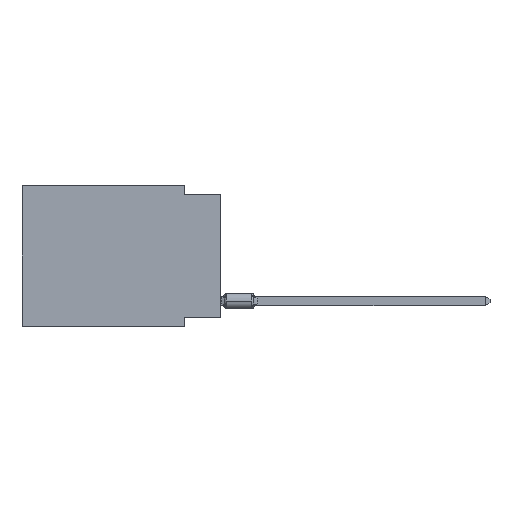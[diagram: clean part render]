
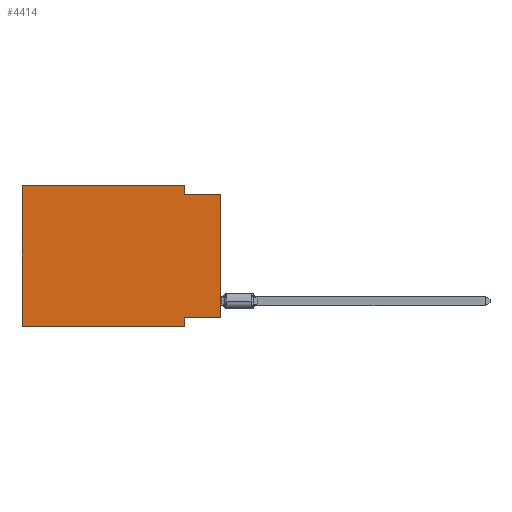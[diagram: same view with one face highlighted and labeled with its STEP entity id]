
A CAD part, left-side view. The second image highlights one B-rep face of the part: STEP entity #4414.
In plain terms, the highlighted planar face has unit normal (-1, 0, 0).
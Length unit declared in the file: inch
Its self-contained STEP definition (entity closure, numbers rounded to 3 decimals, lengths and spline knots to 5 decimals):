
#232 = DIRECTION ( 'NONE',  ( 0., -1., 0. ) ) ;
#452 = ORIENTED_EDGE ( 'NONE', *, *, #15030, .F. ) ;
#1070 = CARTESIAN_POINT ( 'NONE',  ( 0., 0.1, -0.39 ) ) ;
#1318 = LINE ( 'NONE', #1070, #5441 ) ;
#1820 = ORIENTED_EDGE ( 'NONE', *, *, #14614, .F. ) ;
#2452 = CARTESIAN_POINT ( 'NONE',  ( 0., 0., -0.025 ) ) ;
#2698 = LINE ( 'NONE', #4498, #14170 ) ;
#2872 = EDGE_CURVE ( 'NONE', #19427, #13744, #1318, .T. ) ;
#3164 = VECTOR ( 'NONE', #232, 39.37008 ) ;
#3829 = LINE ( 'NONE', #13427, #3164 ) ;
#4414 = ADVANCED_FACE ( 'NONE', ( #11755 ), #19069, .F. ) ;
#4498 = CARTESIAN_POINT ( 'NONE',  ( 0., 0.1, 0. ) ) ;
#4780 = CARTESIAN_POINT ( 'NONE',  ( 0., 0.55, 0. ) ) ;
#4867 = CARTESIAN_POINT ( 'NONE',  ( 0., 0.1, -0.39 ) ) ;
#5154 = EDGE_CURVE ( 'NONE', #9182, #17868, #16870, .T. ) ;
#5441 = VECTOR ( 'NONE', #8392, 39.37008 ) ;
#7120 = ORIENTED_EDGE ( 'NONE', *, *, #2872, .F. ) ;
#8354 = VECTOR ( 'NONE', #10966, 39.37008 ) ;
#8392 = DIRECTION ( 'NONE',  ( 0., 0., -1. ) ) ;
#9182 = VERTEX_POINT ( 'NONE', #14489 ) ;
#9201 = VECTOR ( 'NONE', #18908, 39.37008 ) ;
#9592 = VERTEX_POINT ( 'NONE', #16276 ) ;
#9670 = CARTESIAN_POINT ( 'NONE',  ( 0., 0., 0. ) ) ;
#10638 = EDGE_LOOP ( 'NONE', ( #14295, #13330, #23517, #16822, #1820, #18692, #7120, #452 ) ) ;
#10966 = DIRECTION ( 'NONE',  ( 0., 0., 1. ) ) ;
#11065 = VECTOR ( 'NONE', #11390, 39.37008 ) ;
#11390 = DIRECTION ( 'NONE',  ( 0., 1., 0. ) ) ;
#11427 = EDGE_CURVE ( 'NONE', #9592, #13744, #3829, .T. ) ;
#11755 = FACE_OUTER_BOUND ( 'NONE', #10638, .T. ) ;
#11759 = EDGE_CURVE ( 'NONE', #23703, #17868, #22747, .T. ) ;
#11925 = CARTESIAN_POINT ( 'NONE',  ( 0., 0., -0.025 ) ) ;
#12008 = VERTEX_POINT ( 'NONE', #16710 ) ;
#12633 = LINE ( 'NONE', #16476, #8354 ) ;
#12945 = CARTESIAN_POINT ( 'NONE',  ( 0., 0.55, 0. ) ) ;
#13330 = ORIENTED_EDGE ( 'NONE', *, *, #11759, .F. ) ;
#13383 = DIRECTION ( 'NONE',  ( 0., 0., -1. ) ) ;
#13427 = CARTESIAN_POINT ( 'NONE',  ( 0., 0.55, -0.39 ) ) ;
#13744 = VERTEX_POINT ( 'NONE', #4867 ) ;
#14131 = DIRECTION ( 'NONE',  ( 1., 0., 0. ) ) ;
#14170 = VECTOR ( 'NONE', #13383, 39.37008 ) ;
#14295 = ORIENTED_EDGE ( 'NONE', *, *, #5154, .T. ) ;
#14489 = CARTESIAN_POINT ( 'NONE',  ( 0., 0., -0.365 ) ) ;
#14614 = EDGE_CURVE ( 'NONE', #9592, #16806, #12633, .T. ) ;
#15030 = EDGE_CURVE ( 'NONE', #9182, #19427, #20242, .T. ) ;
#15275 = DIRECTION ( 'NONE',  ( 0., -1., 0. ) ) ;
#15423 = LINE ( 'NONE', #19474, #20814 ) ;
#16276 = CARTESIAN_POINT ( 'NONE',  ( 0., 0.55, -0.39 ) ) ;
#16476 = CARTESIAN_POINT ( 'NONE',  ( 0., 0.55, 0. ) ) ;
#16710 = CARTESIAN_POINT ( 'NONE',  ( 0., 0.1, 0. ) ) ;
#16788 = EDGE_CURVE ( 'NONE', #12008, #23703, #2698, .T. ) ;
#16806 = VERTEX_POINT ( 'NONE', #12945 ) ;
#16822 = ORIENTED_EDGE ( 'NONE', *, *, #22508, .F. ) ;
#16870 = LINE ( 'NONE', #9670, #9201 ) ;
#17354 = DIRECTION ( 'NONE',  ( 0., -1., 0. ) ) ;
#17868 = VERTEX_POINT ( 'NONE', #11925 ) ;
#18692 = ORIENTED_EDGE ( 'NONE', *, *, #11427, .T. ) ;
#18908 = DIRECTION ( 'NONE',  ( 0., 0., 1. ) ) ;
#19069 = PLANE ( 'NONE',  #21841 ) ;
#19427 = VERTEX_POINT ( 'NONE', #21134 ) ;
#19474 = CARTESIAN_POINT ( 'NONE',  ( 0., 0.55, 0. ) ) ;
#20242 = LINE ( 'NONE', #20377, #11065 ) ;
#20377 = CARTESIAN_POINT ( 'NONE',  ( 0., 0., -0.365 ) ) ;
#20814 = VECTOR ( 'NONE', #17354, 39.37008 ) ;
#21134 = CARTESIAN_POINT ( 'NONE',  ( 0., 0.1, -0.365 ) ) ;
#21456 = DIRECTION ( 'NONE',  ( 0., 0., -1. ) ) ;
#21841 = AXIS2_PLACEMENT_3D ( 'NONE', #4780, #14131, #21456 ) ;
#22508 = EDGE_CURVE ( 'NONE', #16806, #12008, #15423, .T. ) ;
#22747 = LINE ( 'NONE', #2452, #23111 ) ;
#23019 = CARTESIAN_POINT ( 'NONE',  ( 0., 0.1, -0.025 ) ) ;
#23111 = VECTOR ( 'NONE', #15275, 39.37008 ) ;
#23517 = ORIENTED_EDGE ( 'NONE', *, *, #16788, .F. ) ;
#23703 = VERTEX_POINT ( 'NONE', #23019 ) ;
